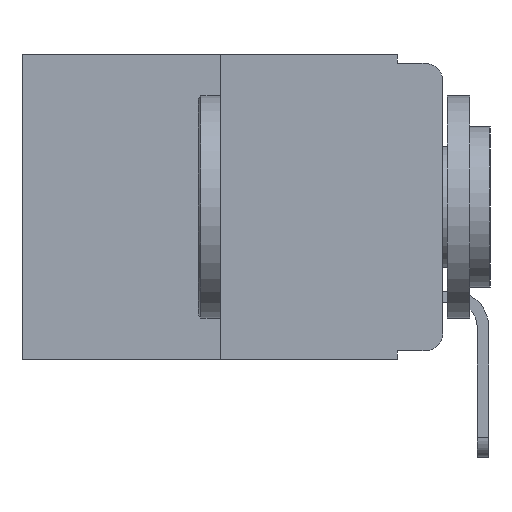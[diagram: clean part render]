
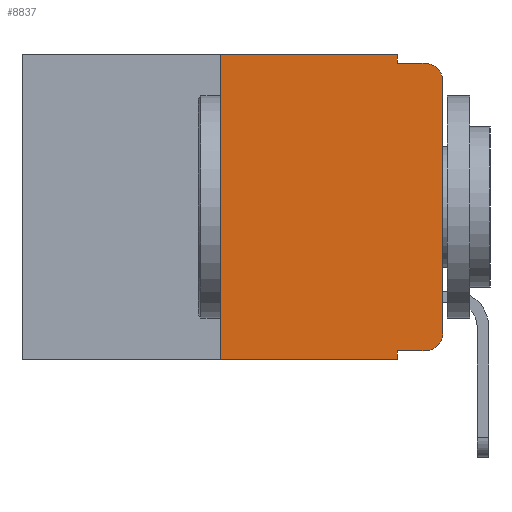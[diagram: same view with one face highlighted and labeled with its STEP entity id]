
A CAD part, left-side view. The second image highlights one B-rep face of the part: STEP entity #8837.
In plain terms, the highlighted planar face has unit normal (-1, 0, 0).
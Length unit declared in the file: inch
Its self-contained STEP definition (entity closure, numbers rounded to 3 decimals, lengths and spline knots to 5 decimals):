
#372 = VERTEX_POINT ( 'NONE', #10433 ) ;
#588 = CARTESIAN_POINT ( 'NONE',  ( 0., 0.473, -0.343 ) ) ;
#1037 = VECTOR ( 'NONE', #8568, 39.37008 ) ;
#1602 = EDGE_CURVE ( 'NONE', #3505, #14961, #9929, .T. ) ;
#1900 = LINE ( 'NONE', #2202, #1037 ) ;
#2134 = DIRECTION ( 'NONE',  ( 0., -1., 0. ) ) ;
#2161 = LINE ( 'NONE', #5064, #13776 ) ;
#2202 = CARTESIAN_POINT ( 'NONE',  ( 0., 0.051, 0. ) ) ;
#2687 = EDGE_CURVE ( 'NONE', #14483, #6152, #7304, .T. ) ;
#2875 = EDGE_CURVE ( 'NONE', #372, #7954, #2161, .T. ) ;
#3428 = CARTESIAN_POINT ( 'NONE',  ( 0., 0.473, 0. ) ) ;
#3505 = VERTEX_POINT ( 'NONE', #18241 ) ;
#3785 = VECTOR ( 'NONE', #7343, 39.37008 ) ;
#4237 = DIRECTION ( 'NONE',  ( 0., 0., 1. ) ) ;
#5064 = CARTESIAN_POINT ( 'NONE',  ( 0., 0.473, 0. ) ) ;
#5077 = DIRECTION ( 'NONE',  ( 0., 0., -1. ) ) ;
#5422 = ORIENTED_EDGE ( 'NONE', *, *, #2875, .F. ) ;
#5577 = EDGE_CURVE ( 'NONE', #17078, #6152, #17821, .T. ) ;
#5588 = ORIENTED_EDGE ( 'NONE', *, *, #2687, .F. ) ;
#5629 = DIRECTION ( 'NONE',  ( 0., -1., 0. ) ) ;
#5778 = DIRECTION ( 'NONE',  ( 0., -1., 0. ) ) ;
#5853 = CARTESIAN_POINT ( 'NONE',  ( 0., 0.02, -0.03 ) ) ;
#6007 = CARTESIAN_POINT ( 'NONE',  ( 0., 0.25, 0. ) ) ;
#6152 = VERTEX_POINT ( 'NONE', #11728 ) ;
#6247 = EDGE_CURVE ( 'NONE', #14961, #12186, #10099, .T. ) ;
#6762 = ORIENTED_EDGE ( 'NONE', *, *, #15980, .F. ) ;
#6913 = DIRECTION ( 'NONE',  ( -1., 0., 0. ) ) ;
#7053 = ORIENTED_EDGE ( 'NONE', *, *, #13179, .F. ) ;
#7156 = LINE ( 'NONE', #588, #15049 ) ;
#7304 = LINE ( 'NONE', #10282, #14315 ) ;
#7343 = DIRECTION ( 'NONE',  ( 0., 0., 1. ) ) ;
#7658 = ORIENTED_EDGE ( 'NONE', *, *, #5577, .T. ) ;
#7954 = VERTEX_POINT ( 'NONE', #17898 ) ;
#8144 = ORIENTED_EDGE ( 'NONE', *, *, #6247, .T. ) ;
#8187 = AXIS2_PLACEMENT_3D ( 'NONE', #3428, #18723, #5077 ) ;
#8225 = VERTEX_POINT ( 'NONE', #11085 ) ;
#8227 = VECTOR ( 'NONE', #18445, 39.37008 ) ;
#8383 = EDGE_CURVE ( 'NONE', #10530, #8225, #7156, .T. ) ;
#8548 = CARTESIAN_POINT ( 'NONE',  ( 0., 0.02, -0.333 ) ) ;
#8568 = DIRECTION ( 'NONE',  ( 0., 0., -1. ) ) ;
#8837 = ADVANCED_FACE ( 'NONE', ( #19026 ), #17484, .F. ) ;
#9649 = VECTOR ( 'NONE', #4237, 39.37008 ) ;
#9716 = CARTESIAN_POINT ( 'NONE',  ( 0., 0.051, -0.01 ) ) ;
#9929 = LINE ( 'NONE', #16118, #15740 ) ;
#10099 = CIRCLE ( 'NONE', #20279, 0.02 ) ;
#10282 = CARTESIAN_POINT ( 'NONE',  ( 0., 0.051, -0.01 ) ) ;
#10433 = CARTESIAN_POINT ( 'NONE',  ( 0., 0.25, 0. ) ) ;
#10530 = VERTEX_POINT ( 'NONE', #19646 ) ;
#10677 = DIRECTION ( 'NONE',  ( -1., 0., 0. ) ) ;
#10778 = ORIENTED_EDGE ( 'NONE', *, *, #8383, .T. ) ;
#11085 = CARTESIAN_POINT ( 'NONE',  ( 0., 0.051, -0.343 ) ) ;
#11093 = CARTESIAN_POINT ( 'NONE',  ( 0., 0., -0.313 ) ) ;
#11304 = CARTESIAN_POINT ( 'NONE',  ( 0., 0., -0.03 ) ) ;
#11465 = ORIENTED_EDGE ( 'NONE', *, *, #15159, .T. ) ;
#11728 = CARTESIAN_POINT ( 'NONE',  ( 0., 0.02, -0.01 ) ) ;
#12105 = DIRECTION ( 'NONE',  ( 0., 0., -1. ) ) ;
#12158 = CARTESIAN_POINT ( 'NONE',  ( 0., 0.051, 0. ) ) ;
#12186 = VERTEX_POINT ( 'NONE', #11093 ) ;
#12888 = EDGE_LOOP ( 'NONE', ( #11465, #7658, #5588, #7053, #5422, #6762, #10778, #17446, #19099, #8144 ) ) ;
#13179 = EDGE_CURVE ( 'NONE', #7954, #14483, #1900, .T. ) ;
#13686 = CARTESIAN_POINT ( 'NONE',  ( 0., 0., 0. ) ) ;
#13776 = VECTOR ( 'NONE', #14302, 39.37008 ) ;
#14302 = DIRECTION ( 'NONE',  ( 0., -1., 0. ) ) ;
#14315 = VECTOR ( 'NONE', #5778, 39.37008 ) ;
#14483 = VERTEX_POINT ( 'NONE', #9716 ) ;
#14961 = VERTEX_POINT ( 'NONE', #8548 ) ;
#15049 = VECTOR ( 'NONE', #5629, 39.37008 ) ;
#15159 = EDGE_CURVE ( 'NONE', #12186, #17078, #16460, .T. ) ;
#15740 = VECTOR ( 'NONE', #2134, 39.37008 ) ;
#15980 = EDGE_CURVE ( 'NONE', #10530, #372, #19975, .T. ) ;
#16118 = CARTESIAN_POINT ( 'NONE',  ( 0., 0.051, -0.333 ) ) ;
#16460 = LINE ( 'NONE', #13686, #9649 ) ;
#16557 = CARTESIAN_POINT ( 'NONE',  ( 0., 0.02, -0.313 ) ) ;
#17078 = VERTEX_POINT ( 'NONE', #11304 ) ;
#17446 = ORIENTED_EDGE ( 'NONE', *, *, #19369, .F. ) ;
#17484 = PLANE ( 'NONE',  #8187 ) ;
#17821 = CIRCLE ( 'NONE', #19454, 0.02 ) ;
#17898 = CARTESIAN_POINT ( 'NONE',  ( 0., 0.051, 0. ) ) ;
#18241 = CARTESIAN_POINT ( 'NONE',  ( 0., 0.051, -0.333 ) ) ;
#18445 = DIRECTION ( 'NONE',  ( 0., 0., -1. ) ) ;
#18723 = DIRECTION ( 'NONE',  ( 1., 0., 0. ) ) ;
#19026 = FACE_OUTER_BOUND ( 'NONE', #12888, .T. ) ;
#19099 = ORIENTED_EDGE ( 'NONE', *, *, #1602, .T. ) ;
#19369 = EDGE_CURVE ( 'NONE', #3505, #8225, #19775, .T. ) ;
#19454 = AXIS2_PLACEMENT_3D ( 'NONE', #5853, #10677, #12105 ) ;
#19636 = DIRECTION ( 'NONE',  ( 0., 0., -1. ) ) ;
#19646 = CARTESIAN_POINT ( 'NONE',  ( 0., 0.25, -0.343 ) ) ;
#19775 = LINE ( 'NONE', #12158, #8227 ) ;
#19975 = LINE ( 'NONE', #6007, #3785 ) ;
#20279 = AXIS2_PLACEMENT_3D ( 'NONE', #16557, #6913, #19636 ) ;
